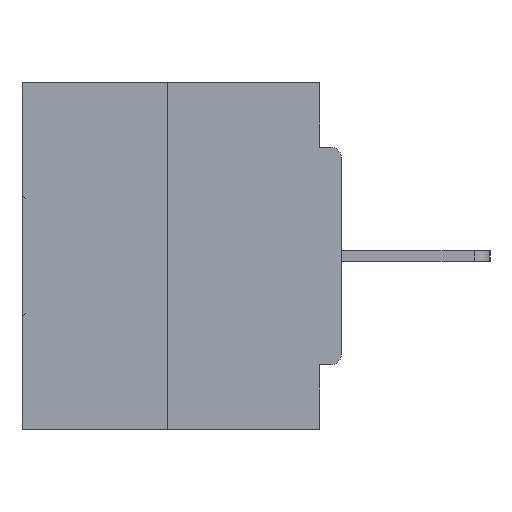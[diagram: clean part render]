
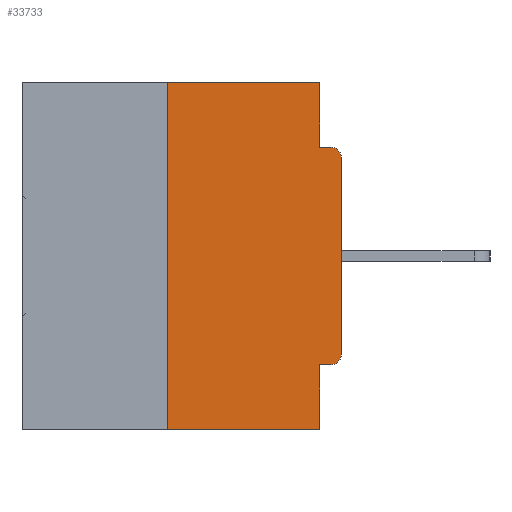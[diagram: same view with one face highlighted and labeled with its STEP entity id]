
A CAD part, left-side view. The second image highlights one B-rep face of the part: STEP entity #33733.
In plain terms, the highlighted planar face has unit normal (-1, 0, 0).
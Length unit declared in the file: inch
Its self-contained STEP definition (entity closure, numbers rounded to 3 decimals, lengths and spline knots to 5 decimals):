
#1531 = CARTESIAN_POINT ( 'NONE',  ( 0., 0.46, -0.5 ) ) ;
#1549 = ORIENTED_EDGE ( 'NONE', *, *, #18012, .F. ) ;
#1744 = CIRCLE ( 'NONE', #26960, 0.015 ) ;
#2601 = CARTESIAN_POINT ( 'NONE',  ( 0., 0., -0.3915 ) ) ;
#3102 = DIRECTION ( 'NONE',  ( 0., -1., 0. ) ) ;
#3450 = CARTESIAN_POINT ( 'NONE',  ( 0., 0.031, -0.4065 ) ) ;
#3720 = ORIENTED_EDGE ( 'NONE', *, *, #20650, .F. ) ;
#3835 = CARTESIAN_POINT ( 'NONE',  ( 0., 0.031, 0. ) ) ;
#4519 = DIRECTION ( 'NONE',  ( 0., -1., 0. ) ) ;
#5031 = LINE ( 'NONE', #8407, #29112 ) ;
#5244 = VERTEX_POINT ( 'NONE', #10789 ) ;
#5267 = VECTOR ( 'NONE', #3102, 39.37008 ) ;
#6215 = CARTESIAN_POINT ( 'NONE',  ( 0., 0.031, -0.5 ) ) ;
#6704 = ORIENTED_EDGE ( 'NONE', *, *, #10563, .T. ) ;
#6909 = LINE ( 'NONE', #32861, #13643 ) ;
#6995 = AXIS2_PLACEMENT_3D ( 'NONE', #37090, #13818, #25300 ) ;
#7060 = CARTESIAN_POINT ( 'NONE',  ( 0., 0.015, -0.0935 ) ) ;
#7423 = VECTOR ( 'NONE', #23499, 39.37008 ) ;
#7616 = VERTEX_POINT ( 'NONE', #35597 ) ;
#8011 = ORIENTED_EDGE ( 'NONE', *, *, #21293, .T. ) ;
#8235 = DIRECTION ( 'NONE',  ( 0., 0., -1. ) ) ;
#8309 = EDGE_CURVE ( 'NONE', #30317, #23152, #16584, .T. ) ;
#8407 = CARTESIAN_POINT ( 'NONE',  ( 0., 0., -0.0935 ) ) ;
#8896 = CARTESIAN_POINT ( 'NONE',  ( 0., 0.25, 0. ) ) ;
#9814 = DIRECTION ( 'NONE',  ( -1., 0., 0. ) ) ;
#10130 = CARTESIAN_POINT ( 'NONE',  ( 0., 0., -0.4065 ) ) ;
#10563 = EDGE_CURVE ( 'NONE', #21934, #15245, #21279, .T. ) ;
#10789 = CARTESIAN_POINT ( 'NONE',  ( 0., 0.031, 0. ) ) ;
#11056 = DIRECTION ( 'NONE',  ( -1., 0., 0. ) ) ;
#11126 = EDGE_CURVE ( 'NONE', #7616, #23621, #5031, .T. ) ;
#11271 = ORIENTED_EDGE ( 'NONE', *, *, #11126, .F. ) ;
#12117 = DIRECTION ( 'NONE',  ( 0., 0., -1. ) ) ;
#12309 = CARTESIAN_POINT ( 'NONE',  ( 0., 0.25, -0.5 ) ) ;
#12381 = DIRECTION ( 'NONE',  ( 0., 0., 1. ) ) ;
#13371 = CARTESIAN_POINT ( 'NONE',  ( 0., 0.015, -0.4065 ) ) ;
#13643 = VECTOR ( 'NONE', #12381, 39.37008 ) ;
#13818 = DIRECTION ( 'NONE',  ( 1., 0., 0. ) ) ;
#14321 = VECTOR ( 'NONE', #12117, 39.37008 ) ;
#15245 = VERTEX_POINT ( 'NONE', #6215 ) ;
#15292 = CARTESIAN_POINT ( 'NONE',  ( 0., 0.015, -0.1085 ) ) ;
#15780 = VECTOR ( 'NONE', #27681, 39.37008 ) ;
#15959 = LINE ( 'NONE', #10130, #33008 ) ;
#16211 = CARTESIAN_POINT ( 'NONE',  ( 0., 0., 0. ) ) ;
#16433 = CIRCLE ( 'NONE', #30846, 0.015 ) ;
#16584 = LINE ( 'NONE', #16211, #15780 ) ;
#16821 = PLANE ( 'NONE',  #6995 ) ;
#17292 = CARTESIAN_POINT ( 'NONE',  ( 0., 0., -0.1085 ) ) ;
#18012 = EDGE_CURVE ( 'NONE', #21934, #30754, #6909, .T. ) ;
#19501 = VERTEX_POINT ( 'NONE', #13371 ) ;
#19881 = ORIENTED_EDGE ( 'NONE', *, *, #30323, .F. ) ;
#20538 = EDGE_CURVE ( 'NONE', #30754, #5244, #36915, .T. ) ;
#20650 = EDGE_CURVE ( 'NONE', #5244, #7616, #32603, .T. ) ;
#20921 = ORIENTED_EDGE ( 'NONE', *, *, #20538, .F. ) ;
#21279 = LINE ( 'NONE', #1531, #28937 ) ;
#21293 = EDGE_CURVE ( 'NONE', #19501, #30317, #1744, .T. ) ;
#21934 = VERTEX_POINT ( 'NONE', #12309 ) ;
#23152 = VERTEX_POINT ( 'NONE', #17292 ) ;
#23499 = DIRECTION ( 'NONE',  ( 0., 0., -1. ) ) ;
#23621 = VERTEX_POINT ( 'NONE', #7060 ) ;
#24863 = CARTESIAN_POINT ( 'NONE',  ( 0., 0.015, -0.3915 ) ) ;
#25300 = DIRECTION ( 'NONE',  ( 0., 0., -1. ) ) ;
#25757 = EDGE_LOOP ( 'NONE', ( #20921, #1549, #6704, #19881, #31562, #8011, #33549, #26656, #11271, #3720 ) ) ;
#26656 = ORIENTED_EDGE ( 'NONE', *, *, #29077, .T. ) ;
#26960 = AXIS2_PLACEMENT_3D ( 'NONE', #24863, #11056, #8235 ) ;
#27681 = DIRECTION ( 'NONE',  ( 0., 0., 1. ) ) ;
#28008 = LINE ( 'NONE', #36987, #7423 ) ;
#28109 = FACE_OUTER_BOUND ( 'NONE', #25757, .T. ) ;
#28161 = DIRECTION ( 'NONE',  ( 0., 1., 0. ) ) ;
#28869 = CARTESIAN_POINT ( 'NONE',  ( 0., 0.46, 0. ) ) ;
#28937 = VECTOR ( 'NONE', #4519, 39.37008 ) ;
#29077 = EDGE_CURVE ( 'NONE', #23152, #23621, #16433, .T. ) ;
#29112 = VECTOR ( 'NONE', #33977, 39.37008 ) ;
#30317 = VERTEX_POINT ( 'NONE', #2601 ) ;
#30323 = EDGE_CURVE ( 'NONE', #30779, #15245, #28008, .T. ) ;
#30754 = VERTEX_POINT ( 'NONE', #8896 ) ;
#30779 = VERTEX_POINT ( 'NONE', #3450 ) ;
#30846 = AXIS2_PLACEMENT_3D ( 'NONE', #15292, #9814, #32752 ) ;
#31562 = ORIENTED_EDGE ( 'NONE', *, *, #35596, .F. ) ;
#32603 = LINE ( 'NONE', #3835, #14321 ) ;
#32752 = DIRECTION ( 'NONE',  ( 0., 0., -1. ) ) ;
#32861 = CARTESIAN_POINT ( 'NONE',  ( 0., 0.25, 0. ) ) ;
#33008 = VECTOR ( 'NONE', #28161, 39.37008 ) ;
#33549 = ORIENTED_EDGE ( 'NONE', *, *, #8309, .T. ) ;
#33733 = ADVANCED_FACE ( 'NONE', ( #28109 ), #16821, .F. ) ;
#33977 = DIRECTION ( 'NONE',  ( 0., -1., 0. ) ) ;
#35596 = EDGE_CURVE ( 'NONE', #19501, #30779, #15959, .T. ) ;
#35597 = CARTESIAN_POINT ( 'NONE',  ( 0., 0.031, -0.0935 ) ) ;
#36915 = LINE ( 'NONE', #28869, #5267 ) ;
#36987 = CARTESIAN_POINT ( 'NONE',  ( 0., 0.031, -0.5 ) ) ;
#37090 = CARTESIAN_POINT ( 'NONE',  ( 0., 0.46, 0. ) ) ;
